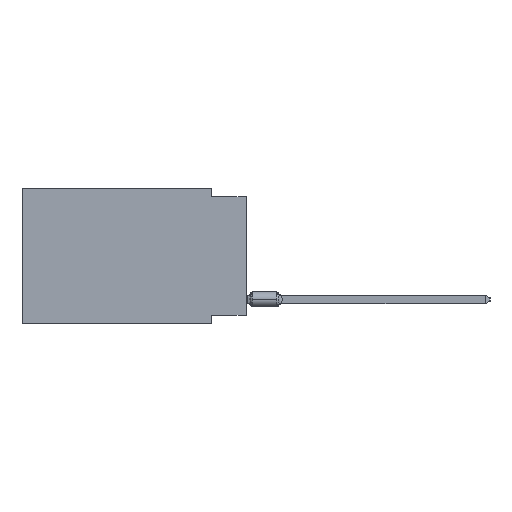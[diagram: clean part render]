
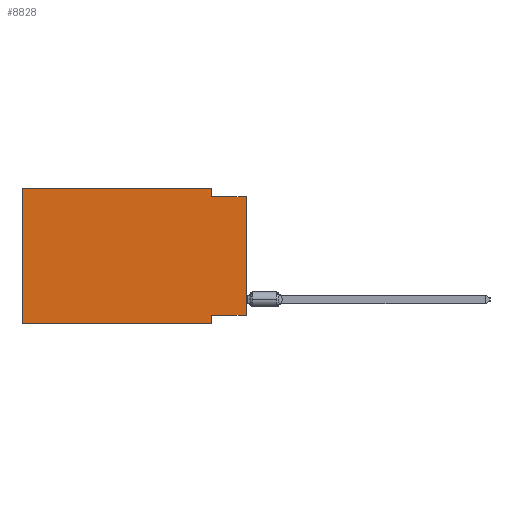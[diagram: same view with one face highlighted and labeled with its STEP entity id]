
A CAD part, left-side view. The second image highlights one B-rep face of the part: STEP entity #8828.
In plain terms, the highlighted planar face has unit normal (-1, 0, 0).
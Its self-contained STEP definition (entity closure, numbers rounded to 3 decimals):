
#1078 = ORIENTED_EDGE ( 'NONE', *, *, #28189, .F. ) ;
#1127 = CARTESIAN_POINT ( 'NONE',  ( 0., 2.54, -0.635 ) ) ;
#2614 = VECTOR ( 'NONE', #12503, 1000. ) ;
#3020 = LINE ( 'NONE', #72516, #15723 ) ;
#5586 = EDGE_CURVE ( 'NONE', #50672, #66947, #73598, .T. ) ;
#6846 = LINE ( 'NONE', #44428, #2614 ) ;
#8828 = ADVANCED_FACE ( 'NONE', ( #20799 ), #32131, .F. ) ;
#9429 = ORIENTED_EDGE ( 'NONE', *, *, #71363, .F. ) ;
#10228 = CARTESIAN_POINT ( 'NONE',  ( 0., 2.54, -9.906 ) ) ;
#11430 = VECTOR ( 'NONE', #78618, 1000. ) ;
#11703 = ORIENTED_EDGE ( 'NONE', *, *, #18457, .T. ) ;
#12503 = DIRECTION ( 'NONE',  ( 0., 1., 0. ) ) ;
#12512 = DIRECTION ( 'NONE',  ( 0., 0., 1. ) ) ;
#12818 = CARTESIAN_POINT ( 'NONE',  ( 0., 16.383, 0. ) ) ;
#12926 = VECTOR ( 'NONE', #12512, 1000. ) ;
#15723 = VECTOR ( 'NONE', #21589, 1000. ) ;
#17501 = ORIENTED_EDGE ( 'NONE', *, *, #51470, .F. ) ;
#18079 = DIRECTION ( 'NONE',  ( 0., -1., 0. ) ) ;
#18180 = EDGE_LOOP ( 'NONE', ( #11703, #48241, #42142, #17501, #64145, #39415, #1078, #9429 ) ) ;
#18457 = EDGE_CURVE ( 'NONE', #53241, #66947, #29509, .T. ) ;
#20392 = DIRECTION ( 'NONE',  ( 1., 0., 0. ) ) ;
#20799 = FACE_OUTER_BOUND ( 'NONE', #18180, .T. ) ;
#21589 = DIRECTION ( 'NONE',  ( 0., 0., -1. ) ) ;
#28189 = EDGE_CURVE ( 'NONE', #64920, #48370, #47007, .T. ) ;
#29301 = LINE ( 'NONE', #53961, #11430 ) ;
#29509 = LINE ( 'NONE', #54163, #12926 ) ;
#29742 = VERTEX_POINT ( 'NONE', #53379 ) ;
#32061 = CARTESIAN_POINT ( 'NONE',  ( 0., 16.383, 0. ) ) ;
#32131 = PLANE ( 'NONE',  #45133 ) ;
#32539 = CARTESIAN_POINT ( 'NONE',  ( 0., 16.383, 0. ) ) ;
#33639 = VERTEX_POINT ( 'NONE', #77966 ) ;
#35656 = LINE ( 'NONE', #53855, #57976 ) ;
#35883 = VECTOR ( 'NONE', #18079, 1000. ) ;
#36272 = LINE ( 'NONE', #12818, #35883 ) ;
#39415 = ORIENTED_EDGE ( 'NONE', *, *, #51812, .T. ) ;
#41750 = DIRECTION ( 'NONE',  ( 0., 0., 1. ) ) ;
#42142 = ORIENTED_EDGE ( 'NONE', *, *, #61205, .F. ) ;
#44107 = CARTESIAN_POINT ( 'NONE',  ( 0., 0., -0.635 ) ) ;
#44428 = CARTESIAN_POINT ( 'NONE',  ( 0., 0., -9.271 ) ) ;
#45133 = AXIS2_PLACEMENT_3D ( 'NONE', #32539, #20392, #49933 ) ;
#47007 = LINE ( 'NONE', #10228, #69713 ) ;
#48241 = ORIENTED_EDGE ( 'NONE', *, *, #5586, .F. ) ;
#48370 = VERTEX_POINT ( 'NONE', #75774 ) ;
#48946 = DIRECTION ( 'NONE',  ( 0., -1., 0. ) ) ;
#49933 = DIRECTION ( 'NONE',  ( 0., 0., -1. ) ) ;
#50672 = VERTEX_POINT ( 'NONE', #1127 ) ;
#51470 = EDGE_CURVE ( 'NONE', #62697, #29742, #36272, .T. ) ;
#51812 = EDGE_CURVE ( 'NONE', #33639, #48370, #29301, .T. ) ;
#51813 = CARTESIAN_POINT ( 'NONE',  ( 0., 2.54, -9.271 ) ) ;
#52019 = CARTESIAN_POINT ( 'NONE',  ( 0., 0., -0.635 ) ) ;
#53241 = VERTEX_POINT ( 'NONE', #64407 ) ;
#53379 = CARTESIAN_POINT ( 'NONE',  ( 0., 2.54, 0. ) ) ;
#53855 = CARTESIAN_POINT ( 'NONE',  ( 0., 16.383, 0. ) ) ;
#53961 = CARTESIAN_POINT ( 'NONE',  ( 0., 16.383, -9.906 ) ) ;
#54163 = CARTESIAN_POINT ( 'NONE',  ( 0., 0., 0. ) ) ;
#57976 = VECTOR ( 'NONE', #41750, 1000. ) ;
#59523 = DIRECTION ( 'NONE',  ( 0., 0., -1. ) ) ;
#61205 = EDGE_CURVE ( 'NONE', #29742, #50672, #3020, .T. ) ;
#62697 = VERTEX_POINT ( 'NONE', #32061 ) ;
#64145 = ORIENTED_EDGE ( 'NONE', *, *, #70870, .F. ) ;
#64407 = CARTESIAN_POINT ( 'NONE',  ( 0., 0., -9.271 ) ) ;
#64920 = VERTEX_POINT ( 'NONE', #51813 ) ;
#66947 = VERTEX_POINT ( 'NONE', #52019 ) ;
#68211 = VECTOR ( 'NONE', #48946, 1000. ) ;
#69713 = VECTOR ( 'NONE', #59523, 1000. ) ;
#70870 = EDGE_CURVE ( 'NONE', #33639, #62697, #35656, .T. ) ;
#71363 = EDGE_CURVE ( 'NONE', #53241, #64920, #6846, .T. ) ;
#72516 = CARTESIAN_POINT ( 'NONE',  ( 0., 2.54, 0. ) ) ;
#73598 = LINE ( 'NONE', #44107, #68211 ) ;
#75774 = CARTESIAN_POINT ( 'NONE',  ( 0., 2.54, -9.906 ) ) ;
#77966 = CARTESIAN_POINT ( 'NONE',  ( 0., 16.383, -9.906 ) ) ;
#78618 = DIRECTION ( 'NONE',  ( 0., -1., 0. ) ) ;
